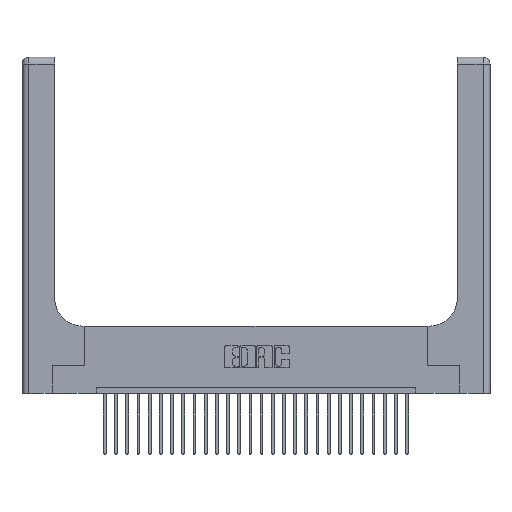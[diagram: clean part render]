
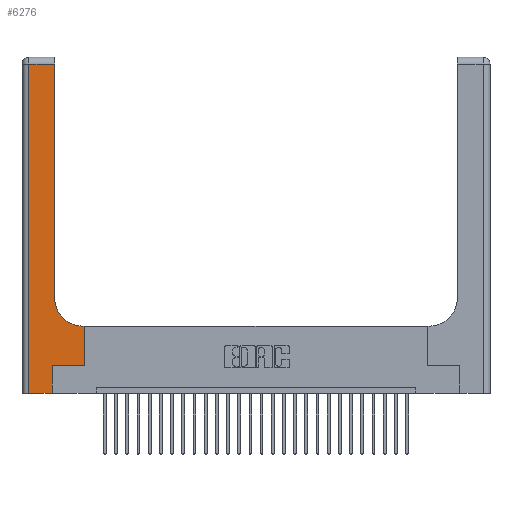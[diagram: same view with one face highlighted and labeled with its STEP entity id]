
A CAD part, top view. The second image highlights one B-rep face of the part: STEP entity #6276.
In plain terms, the highlighted planar face has unit normal (0, 0, 1).
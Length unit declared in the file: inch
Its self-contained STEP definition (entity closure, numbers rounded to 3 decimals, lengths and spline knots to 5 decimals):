
#103 = AXIS2_PLACEMENT_3D ( 'NONE', #17858, #22356, #24754 ) ;
#604 = CARTESIAN_POINT ( 'NONE',  ( 0., 0., 0.37 ) ) ;
#676 = DIRECTION ( 'NONE',  ( 0., -1., 0. ) ) ;
#886 = CARTESIAN_POINT ( 'NONE',  ( 0.2915, 2.94, 0.37 ) ) ;
#1376 = ORIENTED_EDGE ( 'NONE', *, *, #14660, .T. ) ;
#1581 = EDGE_CURVE ( 'NONE', #24178, #16211, #13116, .T. ) ;
#2681 = ORIENTED_EDGE ( 'NONE', *, *, #4002, .T. ) ;
#2791 = DIRECTION ( 'NONE',  ( 0., 1., 0. ) ) ;
#2929 = ORIENTED_EDGE ( 'NONE', *, *, #6430, .T. ) ;
#2945 = VERTEX_POINT ( 'NONE', #16715 ) ;
#3217 = VECTOR ( 'NONE', #18483, 39.37008 ) ;
#3277 = EDGE_CURVE ( 'NONE', #2945, #19334, #11150, .T. ) ;
#3429 = LINE ( 'NONE', #10319, #25898 ) ;
#3978 = VERTEX_POINT ( 'NONE', #886 ) ;
#4002 = EDGE_CURVE ( 'NONE', #19334, #24903, #7291, .T. ) ;
#4367 = LINE ( 'NONE', #16202, #14976 ) ;
#4403 = DIRECTION ( 'NONE',  ( 1., 0., 0. ) ) ;
#4638 = ORIENTED_EDGE ( 'NONE', *, *, #17391, .T. ) ;
#5427 = VECTOR ( 'NONE', #15859, 39.37008 ) ;
#6112 = LINE ( 'NONE', #604, #5427 ) ;
#6276 = ADVANCED_FACE ( 'NONE', ( #13384 ), #13833, .F. ) ;
#6430 = EDGE_CURVE ( 'NONE', #3978, #6637, #9005, .T. ) ;
#6637 = VERTEX_POINT ( 'NONE', #20523 ) ;
#6756 = CARTESIAN_POINT ( 'NONE',  ( 0.2915, 0.6, 0.37 ) ) ;
#6840 = LINE ( 'NONE', #13753, #8239 ) ;
#7291 = CIRCLE ( 'NONE', #103, 0.25 ) ;
#7363 = CARTESIAN_POINT ( 'NONE',  ( 0.269, 0.25, 0.37 ) ) ;
#7773 = AXIS2_PLACEMENT_3D ( 'NONE', #9545, #27411, #22749 ) ;
#7953 = CARTESIAN_POINT ( 'NONE',  ( 0.06, 0., 0.37 ) ) ;
#8058 = CARTESIAN_POINT ( 'NONE',  ( 0.269, 0., 0.37 ) ) ;
#8223 = EDGE_LOOP ( 'NONE', ( #4638, #2929, #13830, #1376, #27942, #8532, #12358, #11740, #2681 ) ) ;
#8239 = VECTOR ( 'NONE', #2791, 39.37008 ) ;
#8381 = EDGE_CURVE ( 'NONE', #16211, #2945, #3429, .T. ) ;
#8532 = ORIENTED_EDGE ( 'NONE', *, *, #1581, .T. ) ;
#8869 = VERTEX_POINT ( 'NONE', #7953 ) ;
#9005 = LINE ( 'NONE', #13622, #3217 ) ;
#9545 = CARTESIAN_POINT ( 'NONE',  ( 0., 3., 0.37 ) ) ;
#10319 = CARTESIAN_POINT ( 'NONE',  ( 0.5585, 0.25, 0.37 ) ) ;
#10930 = DIRECTION ( 'NONE',  ( -1., 0., 0. ) ) ;
#11150 = LINE ( 'NONE', #6756, #27109 ) ;
#11740 = ORIENTED_EDGE ( 'NONE', *, *, #3277, .T. ) ;
#12358 = ORIENTED_EDGE ( 'NONE', *, *, #8381, .T. ) ;
#13116 = LINE ( 'NONE', #20787, #13789 ) ;
#13384 = FACE_OUTER_BOUND ( 'NONE', #8223, .T. ) ;
#13622 = CARTESIAN_POINT ( 'NONE',  ( 0., 2.94, 0.37 ) ) ;
#13753 = CARTESIAN_POINT ( 'NONE',  ( 0.2915, 3., 0.37 ) ) ;
#13789 = VECTOR ( 'NONE', #4403, 39.37008 ) ;
#13830 = ORIENTED_EDGE ( 'NONE', *, *, #19404, .T. ) ;
#13833 = PLANE ( 'NONE',  #7773 ) ;
#14223 = CARTESIAN_POINT ( 'NONE',  ( 0.269, 0., 0.37 ) ) ;
#14660 = EDGE_CURVE ( 'NONE', #8869, #23283, #6112, .T. ) ;
#14976 = VECTOR ( 'NONE', #676, 39.37008 ) ;
#15859 = DIRECTION ( 'NONE',  ( 1., 0., 0. ) ) ;
#16202 = CARTESIAN_POINT ( 'NONE',  ( 0.06, 3., 0.37 ) ) ;
#16211 = VERTEX_POINT ( 'NONE', #21014 ) ;
#16715 = CARTESIAN_POINT ( 'NONE',  ( 0.5585, 0.6, 0.37 ) ) ;
#17391 = EDGE_CURVE ( 'NONE', #24903, #3978, #6840, .T. ) ;
#17858 = CARTESIAN_POINT ( 'NONE',  ( 0.5415, 0.85, 0.37 ) ) ;
#18483 = DIRECTION ( 'NONE',  ( -1., 0., 0. ) ) ;
#19334 = VERTEX_POINT ( 'NONE', #20190 ) ;
#19404 = EDGE_CURVE ( 'NONE', #6637, #8869, #4367, .T. ) ;
#20190 = CARTESIAN_POINT ( 'NONE',  ( 0.5415, 0.6, 0.37 ) ) ;
#20523 = CARTESIAN_POINT ( 'NONE',  ( 0.06, 2.94, 0.37 ) ) ;
#20787 = CARTESIAN_POINT ( 'NONE',  ( 0.269, 0.25, 0.37 ) ) ;
#21014 = CARTESIAN_POINT ( 'NONE',  ( 0.5585, 0.25, 0.37 ) ) ;
#21576 = DIRECTION ( 'NONE',  ( 0., 1., 0. ) ) ;
#22356 = DIRECTION ( 'NONE',  ( 0., 0., -1. ) ) ;
#22749 = DIRECTION ( 'NONE',  ( -1., 0., 0. ) ) ;
#23142 = CARTESIAN_POINT ( 'NONE',  ( 0.2915, 0.85, 0.37 ) ) ;
#23265 = LINE ( 'NONE', #8058, #26997 ) ;
#23283 = VERTEX_POINT ( 'NONE', #14223 ) ;
#23681 = DIRECTION ( 'NONE',  ( 0., 1., 0. ) ) ;
#24178 = VERTEX_POINT ( 'NONE', #7363 ) ;
#24284 = EDGE_CURVE ( 'NONE', #23283, #24178, #23265, .T. ) ;
#24754 = DIRECTION ( 'NONE',  ( 1., 0., 0. ) ) ;
#24903 = VERTEX_POINT ( 'NONE', #23142 ) ;
#25898 = VECTOR ( 'NONE', #23681, 39.37008 ) ;
#26997 = VECTOR ( 'NONE', #21576, 39.37008 ) ;
#27109 = VECTOR ( 'NONE', #10930, 39.37008 ) ;
#27411 = DIRECTION ( 'NONE',  ( 0., 0., -1. ) ) ;
#27942 = ORIENTED_EDGE ( 'NONE', *, *, #24284, .T. ) ;
